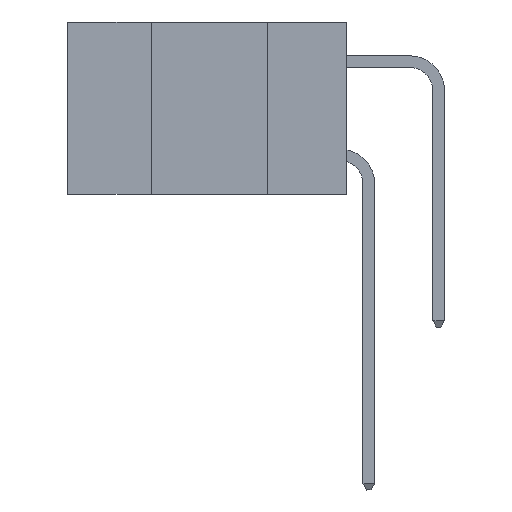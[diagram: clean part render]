
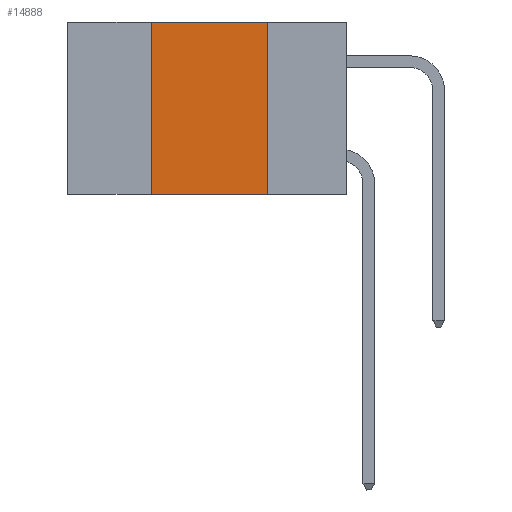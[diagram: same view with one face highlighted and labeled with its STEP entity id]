
A CAD part, left-side view. The second image highlights one B-rep face of the part: STEP entity #14888.
In plain terms, the highlighted planar face has unit normal (-1, 0, 0).
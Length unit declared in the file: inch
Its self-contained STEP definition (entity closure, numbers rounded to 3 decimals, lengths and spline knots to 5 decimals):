
#286 = DIRECTION ( 'NONE',  ( 0., -1., 0. ) ) ;
#535 = CARTESIAN_POINT ( 'NONE',  ( 0., 0.17, 0. ) ) ;
#932 = EDGE_CURVE ( 'NONE', #6200, #16705, #4484, .T. ) ;
#1213 = EDGE_CURVE ( 'NONE', #2389, #6200, #3861, .T. ) ;
#1515 = EDGE_CURVE ( 'NONE', #16705, #9433, #11509, .T. ) ;
#2389 = VERTEX_POINT ( 'NONE', #14959 ) ;
#3020 = DIRECTION ( 'NONE',  ( 0., 0., -1. ) ) ;
#3550 = CARTESIAN_POINT ( 'NONE',  ( 0., 0.17, -0.37 ) ) ;
#3704 = VECTOR ( 'NONE', #11415, 39.37008 ) ;
#3861 = LINE ( 'NONE', #5282, #7749 ) ;
#4215 = VECTOR ( 'NONE', #16807, 39.37008 ) ;
#4344 = ORIENTED_EDGE ( 'NONE', *, *, #6961, .T. ) ;
#4437 = ORIENTED_EDGE ( 'NONE', *, *, #932, .F. ) ;
#4484 = LINE ( 'NONE', #12517, #14014 ) ;
#5068 = ORIENTED_EDGE ( 'NONE', *, *, #1213, .F. ) ;
#5282 = CARTESIAN_POINT ( 'NONE',  ( 0., 0.42, 0. ) ) ;
#6200 = VERTEX_POINT ( 'NONE', #7654 ) ;
#6961 = EDGE_CURVE ( 'NONE', #2389, #9433, #9486, .T. ) ;
#7037 = FACE_OUTER_BOUND ( 'NONE', #10874, .T. ) ;
#7442 = CARTESIAN_POINT ( 'NONE',  ( 0., 0.17, 0. ) ) ;
#7654 = CARTESIAN_POINT ( 'NONE',  ( 0., 0.42, 0. ) ) ;
#7749 = VECTOR ( 'NONE', #13306, 39.37008 ) ;
#9433 = VERTEX_POINT ( 'NONE', #3550 ) ;
#9486 = LINE ( 'NONE', #12592, #4215 ) ;
#9609 = ORIENTED_EDGE ( 'NONE', *, *, #1515, .F. ) ;
#10867 = CARTESIAN_POINT ( 'NONE',  ( 0., 0.6, 0. ) ) ;
#10874 = EDGE_LOOP ( 'NONE', ( #9609, #4437, #5068, #4344 ) ) ;
#11415 = DIRECTION ( 'NONE',  ( 0., 0., -1. ) ) ;
#11509 = LINE ( 'NONE', #535, #3704 ) ;
#12216 = PLANE ( 'NONE',  #12986 ) ;
#12517 = CARTESIAN_POINT ( 'NONE',  ( 0., 0.6, 0. ) ) ;
#12592 = CARTESIAN_POINT ( 'NONE',  ( 0., 0.6, -0.37 ) ) ;
#12986 = AXIS2_PLACEMENT_3D ( 'NONE', #10867, #15258, #3020 ) ;
#13306 = DIRECTION ( 'NONE',  ( 0., 0., 1. ) ) ;
#14014 = VECTOR ( 'NONE', #286, 39.37008 ) ;
#14888 = ADVANCED_FACE ( 'NONE', ( #7037 ), #12216, .F. ) ;
#14959 = CARTESIAN_POINT ( 'NONE',  ( 0., 0.42, -0.37 ) ) ;
#15258 = DIRECTION ( 'NONE',  ( 1., 0., 0. ) ) ;
#16705 = VERTEX_POINT ( 'NONE', #7442 ) ;
#16807 = DIRECTION ( 'NONE',  ( 0., -1., 0. ) ) ;
